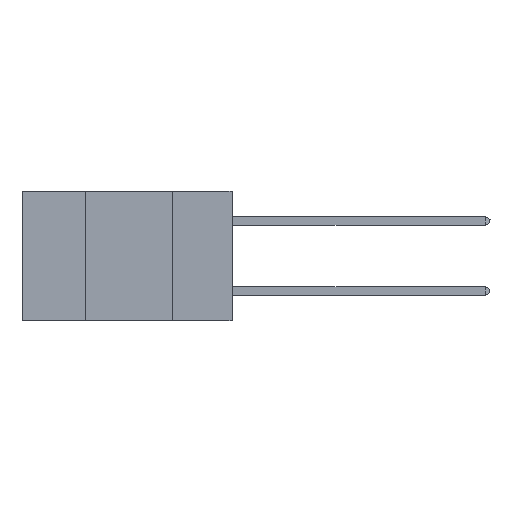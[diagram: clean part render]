
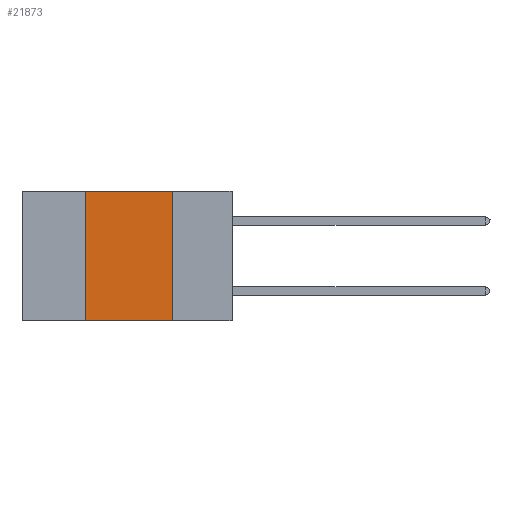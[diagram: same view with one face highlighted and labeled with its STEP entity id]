
A CAD part, left-side view. The second image highlights one B-rep face of the part: STEP entity #21873.
In plain terms, the highlighted planar face has unit normal (-1, 0, 0).
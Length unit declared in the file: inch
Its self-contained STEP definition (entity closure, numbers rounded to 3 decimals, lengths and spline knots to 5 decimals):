
#349 = CARTESIAN_POINT ( 'NONE',  ( 0., 0.6, 0. ) ) ;
#800 = EDGE_CURVE ( 'NONE', #43171, #41173, #4486, .T. ) ;
#4333 = LINE ( 'NONE', #16530, #4673 ) ;
#4486 = LINE ( 'NONE', #349, #18322 ) ;
#4673 = VECTOR ( 'NONE', #19256, 39.37008 ) ;
#5720 = AXIS2_PLACEMENT_3D ( 'NONE', #10032, #47471, #47225 ) ;
#5877 = CARTESIAN_POINT ( 'NONE',  ( 0., 0.6, -0.37 ) ) ;
#6360 = FACE_OUTER_BOUND ( 'NONE', #25308, .T. ) ;
#7451 = EDGE_CURVE ( 'NONE', #17820, #15420, #39386, .T. ) ;
#7899 = DIRECTION ( 'NONE',  ( 0., -1., 0. ) ) ;
#9692 = LINE ( 'NONE', #24619, #22331 ) ;
#10018 = CARTESIAN_POINT ( 'NONE',  ( 0., 0.17, -0.37 ) ) ;
#10032 = CARTESIAN_POINT ( 'NONE',  ( 0., 0.6, 0. ) ) ;
#15275 = ORIENTED_EDGE ( 'NONE', *, *, #7451, .T. ) ;
#15420 = VERTEX_POINT ( 'NONE', #10018 ) ;
#16530 = CARTESIAN_POINT ( 'NONE',  ( 0., 0.42, 0. ) ) ;
#17820 = VERTEX_POINT ( 'NONE', #22404 ) ;
#18322 = VECTOR ( 'NONE', #7899, 39.37008 ) ;
#19256 = DIRECTION ( 'NONE',  ( 0., 0., 1. ) ) ;
#20121 = CARTESIAN_POINT ( 'NONE',  ( 0., 0.17, 0. ) ) ;
#21543 = ORIENTED_EDGE ( 'NONE', *, *, #48283, .F. ) ;
#21873 = ADVANCED_FACE ( 'NONE', ( #6360 ), #32554, .F. ) ;
#22331 = VECTOR ( 'NONE', #35876, 39.37008 ) ;
#22404 = CARTESIAN_POINT ( 'NONE',  ( 0., 0.42, -0.37 ) ) ;
#24619 = CARTESIAN_POINT ( 'NONE',  ( 0., 0.17, 0. ) ) ;
#25308 = EDGE_LOOP ( 'NONE', ( #39650, #37717, #21543, #15275 ) ) ;
#26870 = EDGE_CURVE ( 'NONE', #41173, #15420, #9692, .T. ) ;
#30100 = VECTOR ( 'NONE', #34760, 39.37008 ) ;
#32554 = PLANE ( 'NONE',  #5720 ) ;
#33940 = CARTESIAN_POINT ( 'NONE',  ( 0., 0.42, 0. ) ) ;
#34760 = DIRECTION ( 'NONE',  ( 0., -1., 0. ) ) ;
#35876 = DIRECTION ( 'NONE',  ( 0., 0., -1. ) ) ;
#37717 = ORIENTED_EDGE ( 'NONE', *, *, #800, .F. ) ;
#39386 = LINE ( 'NONE', #5877, #30100 ) ;
#39650 = ORIENTED_EDGE ( 'NONE', *, *, #26870, .F. ) ;
#41173 = VERTEX_POINT ( 'NONE', #20121 ) ;
#43171 = VERTEX_POINT ( 'NONE', #33940 ) ;
#47225 = DIRECTION ( 'NONE',  ( 0., 0., -1. ) ) ;
#47471 = DIRECTION ( 'NONE',  ( 1., 0., 0. ) ) ;
#48283 = EDGE_CURVE ( 'NONE', #17820, #43171, #4333, .T. ) ;
